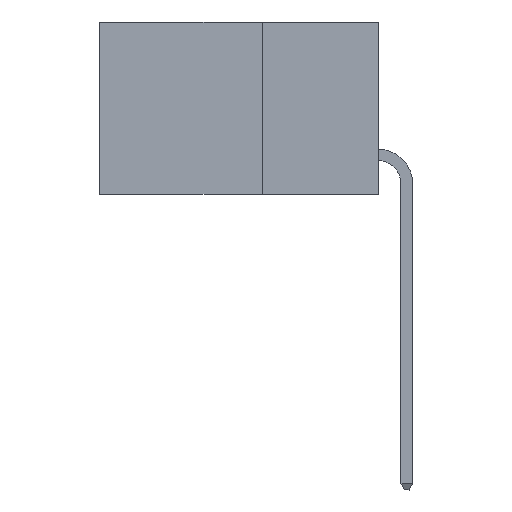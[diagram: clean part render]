
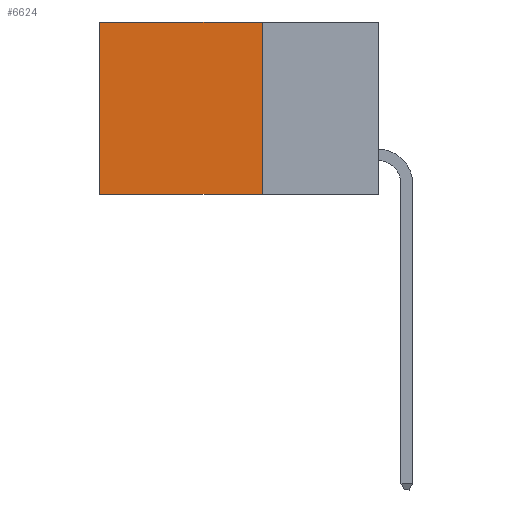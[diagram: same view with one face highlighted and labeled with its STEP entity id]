
A CAD part, left-side view. The second image highlights one B-rep face of the part: STEP entity #6624.
In plain terms, the highlighted planar face has unit normal (-1, 0, 0).
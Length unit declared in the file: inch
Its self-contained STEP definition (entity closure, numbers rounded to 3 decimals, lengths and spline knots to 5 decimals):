
#153 = DIRECTION ( 'NONE',  ( 0., 0., -1. ) ) ;
#477 = VERTEX_POINT ( 'NONE', #10884 ) ;
#515 = CARTESIAN_POINT ( 'NONE',  ( 0.298, 0.25, 0. ) ) ;
#786 = EDGE_CURVE ( 'NONE', #6848, #477, #3742, .T. ) ;
#938 = ORIENTED_EDGE ( 'NONE', *, *, #8790, .F. ) ;
#963 = VERTEX_POINT ( 'NONE', #6147 ) ;
#1638 = DIRECTION ( 'NONE',  ( 0., 0., -1. ) ) ;
#2809 = VERTEX_POINT ( 'NONE', #12205 ) ;
#3205 = FACE_OUTER_BOUND ( 'NONE', #7026, .T. ) ;
#3559 = VECTOR ( 'NONE', #12696, 39.37008 ) ;
#3742 = LINE ( 'NONE', #11595, #9226 ) ;
#4804 = DIRECTION ( 'NONE',  ( 0., 1., 0. ) ) ;
#5036 = AXIS2_PLACEMENT_3D ( 'NONE', #515, #8249, #1638 ) ;
#5160 = CARTESIAN_POINT ( 'NONE',  ( 0.298, 0.25, -0.37 ) ) ;
#6147 = CARTESIAN_POINT ( 'NONE',  ( 0.298, 0.25, -0.37 ) ) ;
#6624 = ADVANCED_FACE ( 'NONE', ( #3205 ), #7103, .F. ) ;
#6655 = DIRECTION ( 'NONE',  ( 0., 0., -1. ) ) ;
#6684 = ORIENTED_EDGE ( 'NONE', *, *, #11408, .T. ) ;
#6848 = VERTEX_POINT ( 'NONE', #13178 ) ;
#7026 = EDGE_LOOP ( 'NONE', ( #6684, #938, #9598, #7333 ) ) ;
#7103 = PLANE ( 'NONE',  #5036 ) ;
#7303 = VECTOR ( 'NONE', #153, 39.37008 ) ;
#7333 = ORIENTED_EDGE ( 'NONE', *, *, #786, .T. ) ;
#7695 = VECTOR ( 'NONE', #6655, 39.37008 ) ;
#8249 = DIRECTION ( 'NONE',  ( 1., 0., 0. ) ) ;
#8790 = EDGE_CURVE ( 'NONE', #963, #2809, #9376, .T. ) ;
#9226 = VECTOR ( 'NONE', #4804, 39.37008 ) ;
#9376 = LINE ( 'NONE', #5160, #3559 ) ;
#9598 = ORIENTED_EDGE ( 'NONE', *, *, #12673, .F. ) ;
#10000 = CARTESIAN_POINT ( 'NONE',  ( 0.298, 0.25, 0. ) ) ;
#10194 = LINE ( 'NONE', #10000, #7303 ) ;
#10564 = LINE ( 'NONE', #14134, #7695 ) ;
#10884 = CARTESIAN_POINT ( 'NONE',  ( 0.298, 0.6, 0. ) ) ;
#11408 = EDGE_CURVE ( 'NONE', #477, #2809, #10564, .T. ) ;
#11595 = CARTESIAN_POINT ( 'NONE',  ( 0.298, 0.25, 0. ) ) ;
#12205 = CARTESIAN_POINT ( 'NONE',  ( 0.298, 0.6, -0.37 ) ) ;
#12673 = EDGE_CURVE ( 'NONE', #6848, #963, #10194, .T. ) ;
#12696 = DIRECTION ( 'NONE',  ( 0., 1., 0. ) ) ;
#13178 = CARTESIAN_POINT ( 'NONE',  ( 0.298, 0.25, 0. ) ) ;
#14134 = CARTESIAN_POINT ( 'NONE',  ( 0.298, 0.6, 0. ) ) ;
